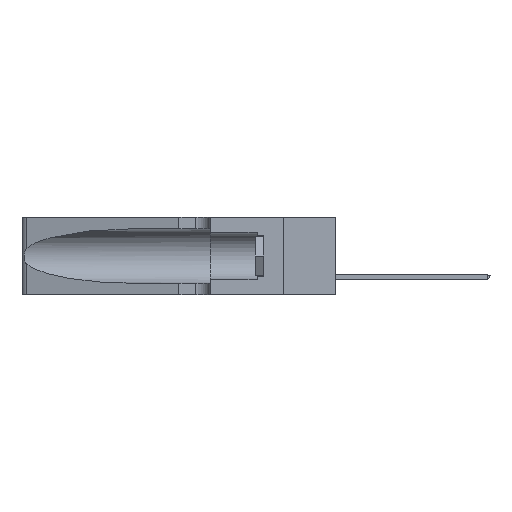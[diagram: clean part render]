
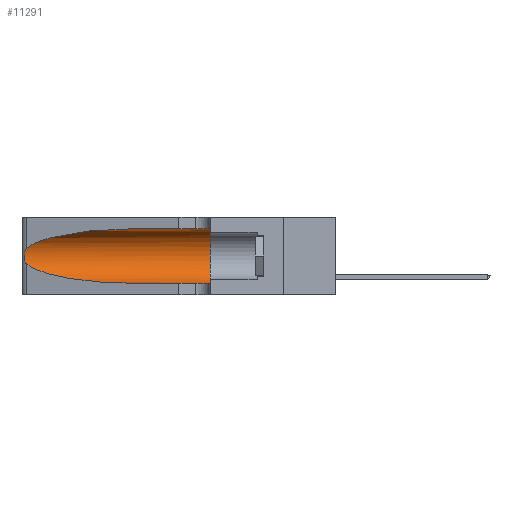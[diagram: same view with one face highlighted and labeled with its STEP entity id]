
A CAD part, left-side view. The second image highlights one B-rep face of the part: STEP entity #11291.
In plain terms, the highlighted cylindrical face has radius 3.308 mm (diameter 6.617 mm), a partial arc.
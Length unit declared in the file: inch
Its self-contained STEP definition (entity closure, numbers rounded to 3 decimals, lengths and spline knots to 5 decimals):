
#304 = B_SPLINE_CURVE_WITH_KNOTS ( 'NONE', 3,
 ( #10904, #27092, #6522, #11106, #15593, #18009, #4158, #22598, #27295, #8694, #24862, #1681, #11205, #27195 ),
 .UNSPECIFIED., .F., .F.,
 ( 4, 2, 2, 2, 2, 2, 4 ),
 ( 0., 0.00027, 0.00053, 0.00107, 0.0016, 0.00187, 0.00214 ),
 .UNSPECIFIED. ) ;
#959 = CARTESIAN_POINT ( 'NONE',  ( 0.1305, 1.61858, 0.31525 ) ) ;
#1263 = EDGE_CURVE ( 'NONE', #13229, #15415, #27165, .T. ) ;
#1616 = CARTESIAN_POINT ( 'NONE',  ( 0.1305, 0.35, 0.185 ) ) ;
#1681 = CARTESIAN_POINT ( 'NONE',  ( 0.25639, 1.23186, 0.15144 ) ) ;
#2162 = EDGE_CURVE ( 'NONE', #26697, #24802, #21820, .T. ) ;
#3061 = ORIENTED_EDGE ( 'NONE', *, *, #2162, .T. ) ;
#3588 = CARTESIAN_POINT ( 'NONE',  ( 0.18966, 0.96281, 0.05475 ) ) ;
#3854 = EDGE_CURVE ( 'NONE', #9606, #12380, #20856, .T. ) ;
#4007 = DIRECTION ( 'NONE',  ( 0., 0., 1. ) ) ;
#4158 = CARTESIAN_POINT ( 'NONE',  ( 0.26075, 1.23896, 0.19203 ) ) ;
#4169 = DIRECTION ( 'NONE',  ( 0., -1., 0. ) ) ;
#4173 = CARTESIAN_POINT ( 'NONE',  ( 0.1305, 0.35, 0.05475 ) ) ;
#4450 = CARTESIAN_POINT ( 'NONE',  ( 0.25487, 1.22718, 0.22369 ) ) ;
#6320 = ORIENTED_EDGE ( 'NONE', *, *, #20650, .T. ) ;
#6522 = CARTESIAN_POINT ( 'NONE',  ( 0.25639, 1.23184, 0.21858 ) ) ;
#7144 = CARTESIAN_POINT ( 'NONE',  ( 0.25487, 1.22718, 0.22369 ) ) ;
#7608 = LINE ( 'NONE', #959, #23407 ) ;
#7963 = EDGE_CURVE ( 'NONE', #26697, #9606, #7608, .T. ) ;
#8602 = CARTESIAN_POINT ( 'NONE',  ( 0.1305, 1.61858, 0.05475 ) ) ;
#8694 = CARTESIAN_POINT ( 'NONE',  ( 0.25856, 1.23593, 0.16098 ) ) ;
#8913 = ORIENTED_EDGE ( 'NONE', *, *, #7963, .F. ) ;
#9115 = CARTESIAN_POINT ( 'NONE',  ( 0.1305, 1.61858, 0.185 ) ) ;
#9606 = VERTEX_POINT ( 'NONE', #9964 ) ;
#9964 = CARTESIAN_POINT ( 'NONE',  ( 0.1305, 0.35, 0.31525 ) ) ;
#10203 = CYLINDRICAL_SURFACE ( 'NONE', #11162, 0.13025 ) ;
#10904 = CARTESIAN_POINT ( 'NONE',  ( 0.25487, 1.22718, 0.22369 ) ) ;
#10977 = FACE_OUTER_BOUND ( 'NONE', #21363, .T. ) ;
#11074 = CARTESIAN_POINT ( 'NONE',  ( 0.25487, 1.22718, 0.14631 ) ) ;
#11106 = CARTESIAN_POINT ( 'NONE',  ( 0.25787, 1.23484, 0.2124 ) ) ;
#11141 = VECTOR ( 'NONE', #4169, 39.37008 ) ;
#11162 = AXIS2_PLACEMENT_3D ( 'NONE', #9115, #16026, #15933 ) ;
#11205 = CARTESIAN_POINT ( 'NONE',  ( 0.25555, 1.22993, 0.14849 ) ) ;
#11291 = ADVANCED_FACE ( 'NONE', ( #10977 ), #10203, .F. ) ;
#12380 = VERTEX_POINT ( 'NONE', #4173 ) ;
#12951 = CARTESIAN_POINT ( 'NONE',  ( 0.25487, 1.22718, 0.14631 ) ) ;
#13062 = ORIENTED_EDGE ( 'NONE', *, *, #3854, .F. ) ;
#13148 = CARTESIAN_POINT ( 'NONE',  ( 0.2373, 1.15595, 0.08982 ) ) ;
#13229 = VERTEX_POINT ( 'NONE', #11074 ) ;
#13536 = ORIENTED_EDGE ( 'NONE', *, *, #22786, .T. ) ;
#14367 = CARTESIAN_POINT ( 'NONE',  ( 0.18966, 0.96281, 0.31525 ) ) ;
#14726 = CARTESIAN_POINT ( 'NONE',  ( 0.1305, 0.72297, 0.31525 ) ) ;
#15389 = CARTESIAN_POINT ( 'NONE',  ( 0.2373, 1.15595, 0.28018 ) ) ;
#15415 = VERTEX_POINT ( 'NONE', #17150 ) ;
#15593 = CARTESIAN_POINT ( 'NONE',  ( 0.25854, 1.2359, 0.20912 ) ) ;
#15933 = DIRECTION ( 'NONE',  ( 0., 0., -1. ) ) ;
#16026 = DIRECTION ( 'NONE',  ( 0., -1., 0. ) ) ;
#17150 = CARTESIAN_POINT ( 'NONE',  ( 0.1305, 0.72297, 0.05475 ) ) ;
#17549 = CARTESIAN_POINT ( 'NONE',  ( 0.1305, 0.72297, 0.05475 ) ) ;
#17812 = AXIS2_PLACEMENT_3D ( 'NONE', #1616, #17860, #4007 ) ;
#17860 = DIRECTION ( 'NONE',  ( 0., 1., 0. ) ) ;
#18009 = CARTESIAN_POINT ( 'NONE',  ( 0.26018, 1.23835, 0.19895 ) ) ;
#18388 = CARTESIAN_POINT ( 'NONE',  ( 0.1305, 0.72297, 0.31525 ) ) ;
#20650 = EDGE_CURVE ( 'NONE', #24802, #13229, #304, .T. ) ;
#20856 = CIRCLE ( 'NONE', #17812, 0.13025 ) ;
#21363 = EDGE_LOOP ( 'NONE', ( #3061, #6320, #22465, #13536, #13062, #8913 ) ) ;
#21820 =( BOUNDED_CURVE ( )  B_SPLINE_CURVE ( 3, ( #14726, #14367, #15389, #4450 ),
 .UNSPECIFIED., .F., .F. ) 
 B_SPLINE_CURVE_WITH_KNOTS ( ( 4, 4 ),
 ( 1.5708, 2.84003 ),
 .UNSPECIFIED. ) 
 CURVE ( )  GEOMETRIC_REPRESENTATION_ITEM ( )  RATIONAL_B_SPLINE_CURVE ( ( 1., 0.87, 0.87, 1. ) ) 
 REPRESENTATION_ITEM ( '' )  );
#22465 = ORIENTED_EDGE ( 'NONE', *, *, #1263, .T. ) ;
#22598 = CARTESIAN_POINT ( 'NONE',  ( 0.26075, 1.23896, 0.178 ) ) ;
#22786 = EDGE_CURVE ( 'NONE', #15415, #12380, #26075, .T. ) ;
#23407 = VECTOR ( 'NONE', #23645, 39.37008 ) ;
#23645 = DIRECTION ( 'NONE',  ( 0., -1., 0. ) ) ;
#24802 = VERTEX_POINT ( 'NONE', #7144 ) ;
#24862 = CARTESIAN_POINT ( 'NONE',  ( 0.25789, 1.23486, 0.15765 ) ) ;
#26075 = LINE ( 'NONE', #8602, #11141 ) ;
#26697 = VERTEX_POINT ( 'NONE', #18388 ) ;
#27092 = CARTESIAN_POINT ( 'NONE',  ( 0.25555, 1.22994, 0.2215 ) ) ;
#27165 =( BOUNDED_CURVE ( )  B_SPLINE_CURVE ( 3, ( #12951, #13148, #3588, #17549 ),
 .UNSPECIFIED., .F., .F. ) 
 B_SPLINE_CURVE_WITH_KNOTS ( ( 4, 4 ),
 ( 3.44316, 4.71239 ),
 .UNSPECIFIED. ) 
 CURVE ( )  GEOMETRIC_REPRESENTATION_ITEM ( )  RATIONAL_B_SPLINE_CURVE ( ( 1., 0.87, 0.87, 1. ) ) 
 REPRESENTATION_ITEM ( '' )  );
#27195 = CARTESIAN_POINT ( 'NONE',  ( 0.25487, 1.22718, 0.14631 ) ) ;
#27295 = CARTESIAN_POINT ( 'NONE',  ( 0.26017, 1.23833, 0.17102 ) ) ;
